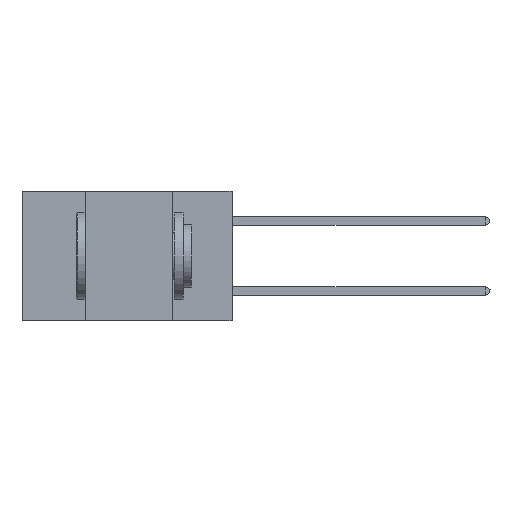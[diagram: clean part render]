
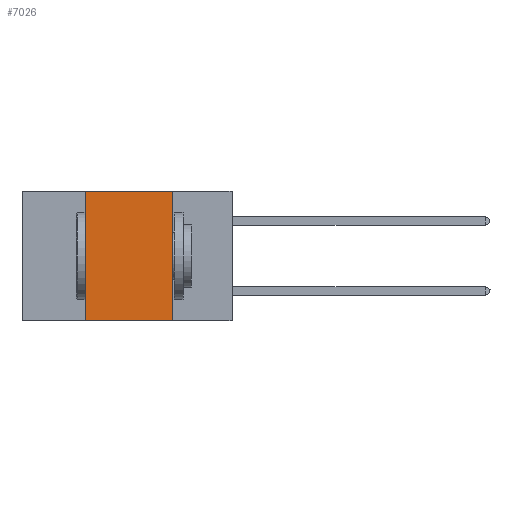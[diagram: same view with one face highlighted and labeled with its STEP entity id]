
A CAD part, left-side view. The second image highlights one B-rep face of the part: STEP entity #7026.
In plain terms, the highlighted planar face has unit normal (-1, 0, 0).
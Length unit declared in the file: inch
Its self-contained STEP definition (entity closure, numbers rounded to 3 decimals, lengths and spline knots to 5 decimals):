
#843 = EDGE_CURVE ( 'NONE', #4012, #16810, #9408, .T. ) ;
#1133 = EDGE_LOOP ( 'NONE', ( #15111, #7528, #15348, #12973 ) ) ;
#1153 = DIRECTION ( 'NONE',  ( 0., 0., -1. ) ) ;
#1903 = LINE ( 'NONE', #11728, #12591 ) ;
#3402 = DIRECTION ( 'NONE',  ( 0., -1., 0. ) ) ;
#4012 = VERTEX_POINT ( 'NONE', #6126 ) ;
#4475 = LINE ( 'NONE', #8194, #12264 ) ;
#4977 = EDGE_CURVE ( 'NONE', #7416, #4012, #15493, .T. ) ;
#5644 = FACE_OUTER_BOUND ( 'NONE', #1133, .T. ) ;
#5699 = VECTOR ( 'NONE', #14825, 39.37008 ) ;
#6126 = CARTESIAN_POINT ( 'NONE',  ( 0., 0.42, 0. ) ) ;
#6150 = CARTESIAN_POINT ( 'NONE',  ( 0., 0.17, 0. ) ) ;
#6189 = DIRECTION ( 'NONE',  ( 0., 0., -1. ) ) ;
#7026 = ADVANCED_FACE ( 'NONE', ( #5644 ), #10370, .F. ) ;
#7416 = VERTEX_POINT ( 'NONE', #8043 ) ;
#7528 = ORIENTED_EDGE ( 'NONE', *, *, #843, .F. ) ;
#8043 = CARTESIAN_POINT ( 'NONE',  ( 0., 0.42, -0.37 ) ) ;
#8194 = CARTESIAN_POINT ( 'NONE',  ( 0., 0.17, 0. ) ) ;
#8593 = AXIS2_PLACEMENT_3D ( 'NONE', #13127, #14510, #6189 ) ;
#9056 = EDGE_CURVE ( 'NONE', #7416, #15593, #1903, .T. ) ;
#9408 = LINE ( 'NONE', #15103, #5699 ) ;
#9829 = DIRECTION ( 'NONE',  ( 0., 0., 1. ) ) ;
#10370 = PLANE ( 'NONE',  #8593 ) ;
#11728 = CARTESIAN_POINT ( 'NONE',  ( 0., 0.6, -0.37 ) ) ;
#11832 = VECTOR ( 'NONE', #9829, 39.37008 ) ;
#12067 = EDGE_CURVE ( 'NONE', #16810, #15593, #4475, .T. ) ;
#12264 = VECTOR ( 'NONE', #1153, 39.37008 ) ;
#12591 = VECTOR ( 'NONE', #3402, 39.37008 ) ;
#12973 = ORIENTED_EDGE ( 'NONE', *, *, #9056, .T. ) ;
#13127 = CARTESIAN_POINT ( 'NONE',  ( 0., 0.6, 0. ) ) ;
#14510 = DIRECTION ( 'NONE',  ( 1., 0., 0. ) ) ;
#14825 = DIRECTION ( 'NONE',  ( 0., -1., 0. ) ) ;
#15103 = CARTESIAN_POINT ( 'NONE',  ( 0., 0.6, 0. ) ) ;
#15111 = ORIENTED_EDGE ( 'NONE', *, *, #12067, .F. ) ;
#15348 = ORIENTED_EDGE ( 'NONE', *, *, #4977, .F. ) ;
#15493 = LINE ( 'NONE', #16645, #11832 ) ;
#15593 = VERTEX_POINT ( 'NONE', #16289 ) ;
#16289 = CARTESIAN_POINT ( 'NONE',  ( 0., 0.17, -0.37 ) ) ;
#16645 = CARTESIAN_POINT ( 'NONE',  ( 0., 0.42, 0. ) ) ;
#16810 = VERTEX_POINT ( 'NONE', #6150 ) ;
